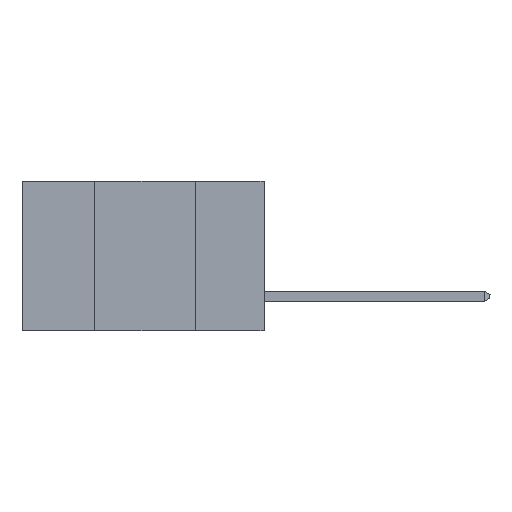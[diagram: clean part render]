
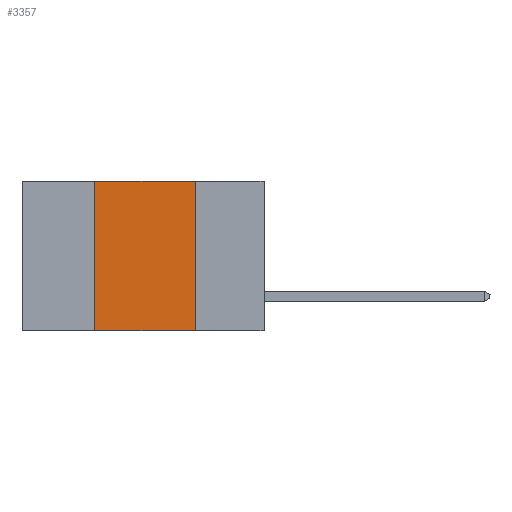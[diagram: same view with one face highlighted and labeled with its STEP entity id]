
A CAD part, left-side view. The second image highlights one B-rep face of the part: STEP entity #3357.
In plain terms, the highlighted planar face has unit normal (-1, 0, 0).
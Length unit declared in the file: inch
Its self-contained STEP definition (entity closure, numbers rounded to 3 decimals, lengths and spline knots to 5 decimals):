
#280 = VERTEX_POINT ( 'NONE', #9190 ) ;
#357 = CARTESIAN_POINT ( 'NONE',  ( 0., 0.42, 0. ) ) ;
#531 = DIRECTION ( 'NONE',  ( 0., 0., -1. ) ) ;
#559 = VERTEX_POINT ( 'NONE', #1107 ) ;
#862 = LINE ( 'NONE', #10295, #7581 ) ;
#1104 = DIRECTION ( 'NONE',  ( 0., 0., -1. ) ) ;
#1107 = CARTESIAN_POINT ( 'NONE',  ( 0., 0.17, 0. ) ) ;
#1487 = FACE_OUTER_BOUND ( 'NONE', #9083, .T. ) ;
#1667 = VECTOR ( 'NONE', #10050, 39.37008 ) ;
#2265 = VECTOR ( 'NONE', #3093, 39.37008 ) ;
#2808 = EDGE_CURVE ( 'NONE', #559, #280, #862, .T. ) ;
#3093 = DIRECTION ( 'NONE',  ( 0., -1., 0. ) ) ;
#3225 = EDGE_CURVE ( 'NONE', #5660, #280, #5297, .T. ) ;
#3357 = ADVANCED_FACE ( 'NONE', ( #1487 ), #5972, .F. ) ;
#3373 = ORIENTED_EDGE ( 'NONE', *, *, #3225, .T. ) ;
#4632 = CARTESIAN_POINT ( 'NONE',  ( 0., 0.6, -0.37 ) ) ;
#4990 = CARTESIAN_POINT ( 'NONE',  ( 0., 0.6, 0. ) ) ;
#5297 = LINE ( 'NONE', #4632, #2265 ) ;
#5420 = VERTEX_POINT ( 'NONE', #7694 ) ;
#5660 = VERTEX_POINT ( 'NONE', #10506 ) ;
#5878 = DIRECTION ( 'NONE',  ( 0., -1., 0. ) ) ;
#5942 = DIRECTION ( 'NONE',  ( 1., 0., 0. ) ) ;
#5972 = PLANE ( 'NONE',  #8411 ) ;
#6169 = EDGE_CURVE ( 'NONE', #5660, #5420, #7914, .T. ) ;
#6447 = VECTOR ( 'NONE', #5878, 39.37008 ) ;
#7185 = ORIENTED_EDGE ( 'NONE', *, *, #2808, .F. ) ;
#7581 = VECTOR ( 'NONE', #531, 39.37008 ) ;
#7694 = CARTESIAN_POINT ( 'NONE',  ( 0., 0.42, 0. ) ) ;
#7914 = LINE ( 'NONE', #357, #1667 ) ;
#8385 = LINE ( 'NONE', #4990, #6447 ) ;
#8411 = AXIS2_PLACEMENT_3D ( 'NONE', #9137, #5942, #1104 ) ;
#8929 = EDGE_CURVE ( 'NONE', #5420, #559, #8385, .T. ) ;
#9083 = EDGE_LOOP ( 'NONE', ( #7185, #10490, #10198, #3373 ) ) ;
#9137 = CARTESIAN_POINT ( 'NONE',  ( 0., 0.6, 0. ) ) ;
#9190 = CARTESIAN_POINT ( 'NONE',  ( 0., 0.17, -0.37 ) ) ;
#10050 = DIRECTION ( 'NONE',  ( 0., 0., 1. ) ) ;
#10198 = ORIENTED_EDGE ( 'NONE', *, *, #6169, .F. ) ;
#10295 = CARTESIAN_POINT ( 'NONE',  ( 0., 0.17, 0. ) ) ;
#10490 = ORIENTED_EDGE ( 'NONE', *, *, #8929, .F. ) ;
#10506 = CARTESIAN_POINT ( 'NONE',  ( 0., 0.42, -0.37 ) ) ;
